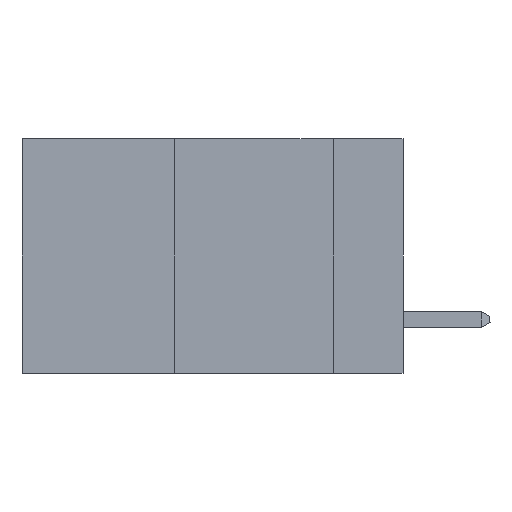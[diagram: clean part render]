
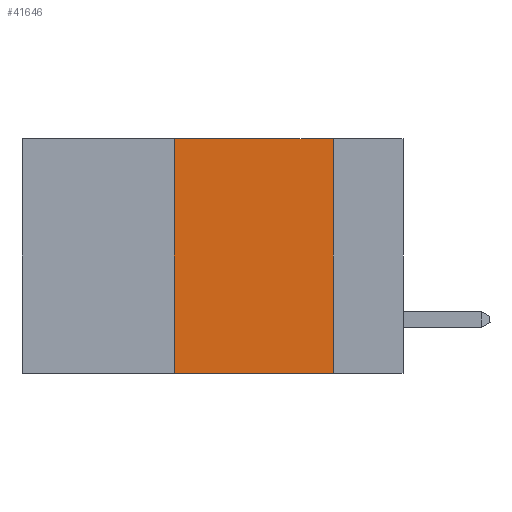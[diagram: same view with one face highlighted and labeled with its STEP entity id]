
A CAD part, left-side view. The second image highlights one B-rep face of the part: STEP entity #41646.
In plain terms, the highlighted planar face has unit normal (-1, 0, 0).
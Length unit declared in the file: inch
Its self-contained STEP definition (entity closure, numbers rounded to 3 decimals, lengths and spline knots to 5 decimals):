
#847 = VECTOR ( 'NONE', #42649, 39.37008 ) ;
#1950 = LINE ( 'NONE', #13621, #41339 ) ;
#2312 = CARTESIAN_POINT ( 'NONE',  ( 0., 0.6, 0. ) ) ;
#2612 = ORIENTED_EDGE ( 'NONE', *, *, #3105, .T. ) ;
#3105 = EDGE_CURVE ( 'NONE', #26545, #44797, #1950, .T. ) ;
#4762 = DIRECTION ( 'NONE',  ( 0., 0., -1. ) ) ;
#5113 = EDGE_LOOP ( 'NONE', ( #34695, #45308, #27532, #2612 ) ) ;
#5793 = CARTESIAN_POINT ( 'NONE',  ( 0., 0.6, 0. ) ) ;
#5905 = VECTOR ( 'NONE', #4762, 39.37008 ) ;
#11248 = EDGE_CURVE ( 'NONE', #13050, #44797, #35313, .T. ) ;
#13050 = VERTEX_POINT ( 'NONE', #29927 ) ;
#13621 = CARTESIAN_POINT ( 'NONE',  ( 0., 0.6, -0.37 ) ) ;
#16460 = DIRECTION ( 'NONE',  ( 0., -1., 0. ) ) ;
#16515 = DIRECTION ( 'NONE',  ( 1., 0., 0. ) ) ;
#17668 = EDGE_CURVE ( 'NONE', #34742, #13050, #38274, .T. ) ;
#20664 = CARTESIAN_POINT ( 'NONE',  ( 0., 0.36, -0.37 ) ) ;
#21852 = CARTESIAN_POINT ( 'NONE',  ( 0., 0.11, 0. ) ) ;
#24761 = AXIS2_PLACEMENT_3D ( 'NONE', #5793, #16515, #27385 ) ;
#26545 = VERTEX_POINT ( 'NONE', #20664 ) ;
#27068 = PLANE ( 'NONE',  #24761 ) ;
#27385 = DIRECTION ( 'NONE',  ( 0., 0., -1. ) ) ;
#27532 = ORIENTED_EDGE ( 'NONE', *, *, #35992, .F. ) ;
#29184 = DIRECTION ( 'NONE',  ( 0., -1., 0. ) ) ;
#29808 = LINE ( 'NONE', #35569, #847 ) ;
#29927 = CARTESIAN_POINT ( 'NONE',  ( 0., 0.11, 0. ) ) ;
#34695 = ORIENTED_EDGE ( 'NONE', *, *, #11248, .F. ) ;
#34742 = VERTEX_POINT ( 'NONE', #38775 ) ;
#35313 = LINE ( 'NONE', #21852, #5905 ) ;
#35569 = CARTESIAN_POINT ( 'NONE',  ( 0., 0.36, 0. ) ) ;
#35992 = EDGE_CURVE ( 'NONE', #26545, #34742, #29808, .T. ) ;
#36014 = VECTOR ( 'NONE', #16460, 39.37008 ) ;
#38274 = LINE ( 'NONE', #2312, #36014 ) ;
#38775 = CARTESIAN_POINT ( 'NONE',  ( 0., 0.36, 0. ) ) ;
#38908 = FACE_OUTER_BOUND ( 'NONE', #5113, .T. ) ;
#39578 = CARTESIAN_POINT ( 'NONE',  ( 0., 0.11, -0.37 ) ) ;
#41339 = VECTOR ( 'NONE', #29184, 39.37008 ) ;
#41646 = ADVANCED_FACE ( 'NONE', ( #38908 ), #27068, .F. ) ;
#42649 = DIRECTION ( 'NONE',  ( 0., 0., 1. ) ) ;
#44797 = VERTEX_POINT ( 'NONE', #39578 ) ;
#45308 = ORIENTED_EDGE ( 'NONE', *, *, #17668, .F. ) ;
